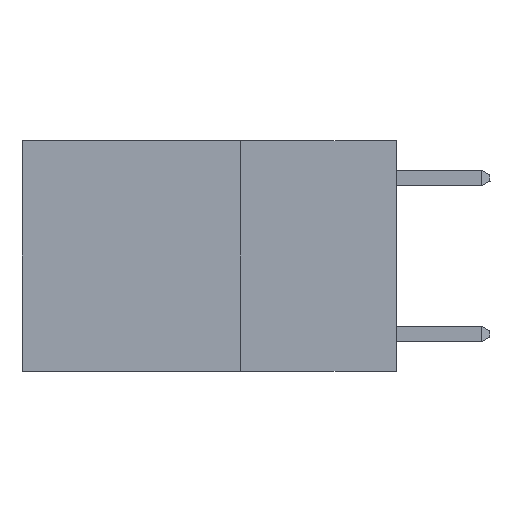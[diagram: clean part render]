
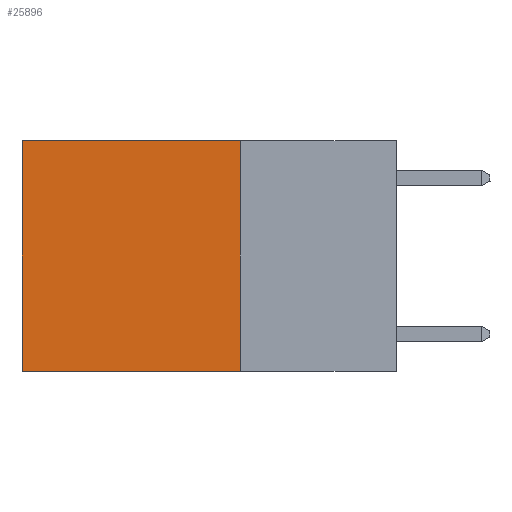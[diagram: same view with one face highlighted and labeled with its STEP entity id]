
A CAD part, left-side view. The second image highlights one B-rep face of the part: STEP entity #25896.
In plain terms, the highlighted planar face has unit normal (-1, 0, 0).
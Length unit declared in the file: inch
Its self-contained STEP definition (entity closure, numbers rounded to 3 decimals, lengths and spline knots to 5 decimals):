
#497 = VERTEX_POINT ( 'NONE', #26025 ) ;
#732 = ORIENTED_EDGE ( 'NONE', *, *, #15469, .F. ) ;
#974 = DIRECTION ( 'NONE',  ( 0., 0., -1. ) ) ;
#1515 = DIRECTION ( 'NONE',  ( 0., 0., -1. ) ) ;
#1625 = DIRECTION ( 'NONE',  ( 1., 0., 0. ) ) ;
#3185 = ORIENTED_EDGE ( 'NONE', *, *, #22381, .F. ) ;
#3721 = CARTESIAN_POINT ( 'NONE',  ( 0.2625, 0.25, 0. ) ) ;
#4279 = VERTEX_POINT ( 'NONE', #19878 ) ;
#5711 = EDGE_LOOP ( 'NONE', ( #14008, #3185, #732, #12061 ) ) ;
#7813 = VECTOR ( 'NONE', #974, 39.37008 ) ;
#7971 = PLANE ( 'NONE',  #14244 ) ;
#8403 = VECTOR ( 'NONE', #23985, 39.37008 ) ;
#8534 = LINE ( 'NONE', #11583, #7813 ) ;
#9189 = CARTESIAN_POINT ( 'NONE',  ( 0.2625, 0.6, -0.37 ) ) ;
#9851 = DIRECTION ( 'NONE',  ( 0., 1., 0. ) ) ;
#9948 = CARTESIAN_POINT ( 'NONE',  ( 0.2625, 0.6, 0. ) ) ;
#10848 = FACE_OUTER_BOUND ( 'NONE', #5711, .T. ) ;
#11583 = CARTESIAN_POINT ( 'NONE',  ( 0.2625, 0.25, 0. ) ) ;
#11833 = VERTEX_POINT ( 'NONE', #15322 ) ;
#12061 = ORIENTED_EDGE ( 'NONE', *, *, #28091, .T. ) ;
#14008 = ORIENTED_EDGE ( 'NONE', *, *, #17859, .T. ) ;
#14244 = AXIS2_PLACEMENT_3D ( 'NONE', #3721, #1625, #16529 ) ;
#14310 = CARTESIAN_POINT ( 'NONE',  ( 0.2625, 0.25, -0.37 ) ) ;
#15322 = CARTESIAN_POINT ( 'NONE',  ( 0.2625, 0.25, -0.37 ) ) ;
#15469 = EDGE_CURVE ( 'NONE', #4279, #11833, #8534, .T. ) ;
#16529 = DIRECTION ( 'NONE',  ( 0., 0., -1. ) ) ;
#16863 = LINE ( 'NONE', #14310, #20967 ) ;
#17859 = EDGE_CURVE ( 'NONE', #497, #19363, #18172, .T. ) ;
#18172 = LINE ( 'NONE', #9948, #20562 ) ;
#19363 = VERTEX_POINT ( 'NONE', #9189 ) ;
#19878 = CARTESIAN_POINT ( 'NONE',  ( 0.2625, 0.25, 0. ) ) ;
#20562 = VECTOR ( 'NONE', #1515, 39.37008 ) ;
#20967 = VECTOR ( 'NONE', #9851, 39.37008 ) ;
#21521 = CARTESIAN_POINT ( 'NONE',  ( 0.2625, 0.25, 0. ) ) ;
#22381 = EDGE_CURVE ( 'NONE', #11833, #19363, #16863, .T. ) ;
#23985 = DIRECTION ( 'NONE',  ( 0., 1., 0. ) ) ;
#25896 = ADVANCED_FACE ( 'NONE', ( #10848 ), #7971, .F. ) ;
#26025 = CARTESIAN_POINT ( 'NONE',  ( 0.2625, 0.6, 0. ) ) ;
#26044 = LINE ( 'NONE', #21521, #8403 ) ;
#28091 = EDGE_CURVE ( 'NONE', #4279, #497, #26044, .T. ) ;
